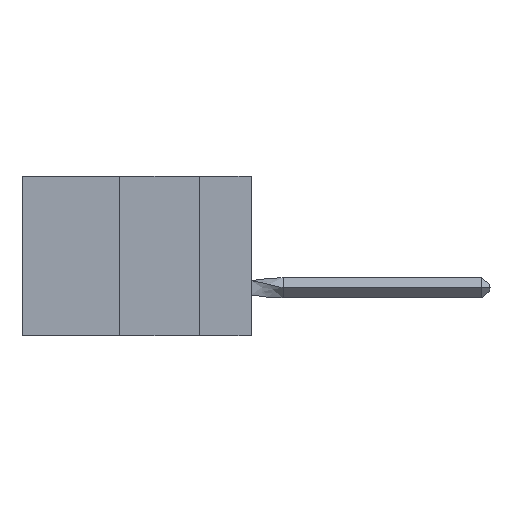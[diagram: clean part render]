
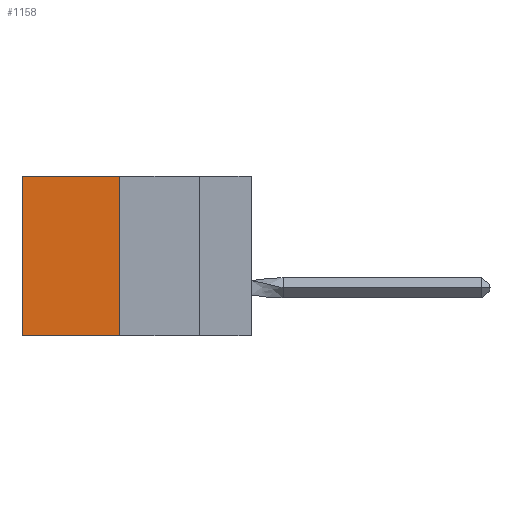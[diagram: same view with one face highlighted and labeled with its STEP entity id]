
A CAD part, left-side view. The second image highlights one B-rep face of the part: STEP entity #1158.
In plain terms, the highlighted planar face has unit normal (-1, 0, 0).
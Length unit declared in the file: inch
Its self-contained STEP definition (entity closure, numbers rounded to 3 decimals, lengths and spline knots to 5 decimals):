
#399 = FACE_OUTER_BOUND ( 'NONE', #5356, .T. ) ;
#806 = EDGE_CURVE ( 'NONE', #8549, #3372, #3013, .T. ) ;
#1036 = CARTESIAN_POINT ( 'NONE',  ( 0.305, 0.413, 0. ) ) ;
#1158 = ADVANCED_FACE ( 'NONE', ( #399 ), #13227, .F. ) ;
#3013 = LINE ( 'NONE', #13089, #9681 ) ;
#3314 = CARTESIAN_POINT ( 'NONE',  ( 0.305, 0.413, -0.5 ) ) ;
#3372 = VERTEX_POINT ( 'NONE', #13958 ) ;
#4151 = CARTESIAN_POINT ( 'NONE',  ( 0.305, 0.72, -0.5 ) ) ;
#4167 = ORIENTED_EDGE ( 'NONE', *, *, #10977, .T. ) ;
#4389 = LINE ( 'NONE', #10302, #15460 ) ;
#4839 = DIRECTION ( 'NONE',  ( 0., 1., 0. ) ) ;
#5128 = DIRECTION ( 'NONE',  ( 1., 0., 0. ) ) ;
#5356 = EDGE_LOOP ( 'NONE', ( #7689, #7182, #9761, #4167 ) ) ;
#5945 = EDGE_CURVE ( 'NONE', #10348, #3372, #10501, .T. ) ;
#7182 = ORIENTED_EDGE ( 'NONE', *, *, #806, .F. ) ;
#7689 = ORIENTED_EDGE ( 'NONE', *, *, #5945, .T. ) ;
#8549 = VERTEX_POINT ( 'NONE', #21183 ) ;
#9681 = VECTOR ( 'NONE', #4839, 39.37008 ) ;
#9761 = ORIENTED_EDGE ( 'NONE', *, *, #20756, .F. ) ;
#9988 = AXIS2_PLACEMENT_3D ( 'NONE', #3314, #5128, #16619 ) ;
#10302 = CARTESIAN_POINT ( 'NONE',  ( 0.305, 0.413, -0.5 ) ) ;
#10348 = VERTEX_POINT ( 'NONE', #10475 ) ;
#10475 = CARTESIAN_POINT ( 'NONE',  ( 0.305, 0.72, 0. ) ) ;
#10501 = LINE ( 'NONE', #4151, #13860 ) ;
#10794 = DIRECTION ( 'NONE',  ( 0., 0., -1. ) ) ;
#10977 = EDGE_CURVE ( 'NONE', #11019, #10348, #16509, .T. ) ;
#11019 = VERTEX_POINT ( 'NONE', #12399 ) ;
#11350 = VECTOR ( 'NONE', #12470, 39.37008 ) ;
#12399 = CARTESIAN_POINT ( 'NONE',  ( 0.305, 0.413, 0. ) ) ;
#12470 = DIRECTION ( 'NONE',  ( 0., 1., 0. ) ) ;
#13089 = CARTESIAN_POINT ( 'NONE',  ( 0.305, 0.413, -0.5 ) ) ;
#13227 = PLANE ( 'NONE',  #9988 ) ;
#13860 = VECTOR ( 'NONE', #14290, 39.37008 ) ;
#13958 = CARTESIAN_POINT ( 'NONE',  ( 0.305, 0.72, -0.5 ) ) ;
#14290 = DIRECTION ( 'NONE',  ( 0., 0., -1. ) ) ;
#15460 = VECTOR ( 'NONE', #10794, 39.37008 ) ;
#16509 = LINE ( 'NONE', #1036, #11350 ) ;
#16619 = DIRECTION ( 'NONE',  ( 0., 0., -1. ) ) ;
#20756 = EDGE_CURVE ( 'NONE', #11019, #8549, #4389, .T. ) ;
#21183 = CARTESIAN_POINT ( 'NONE',  ( 0.305, 0.413, -0.5 ) ) ;
